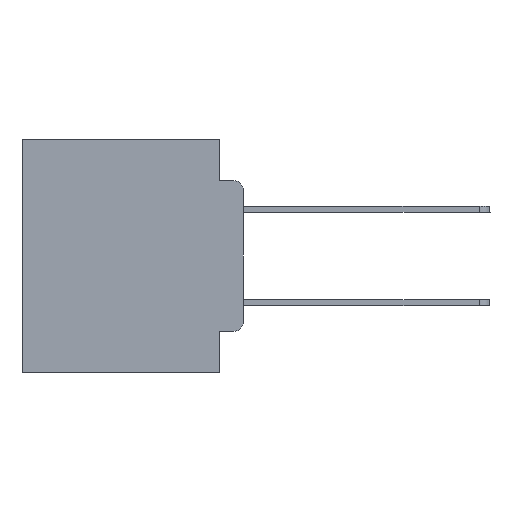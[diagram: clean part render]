
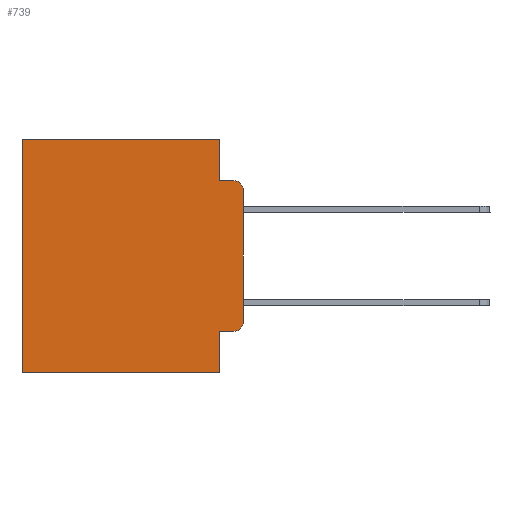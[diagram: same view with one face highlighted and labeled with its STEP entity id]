
A CAD part, left-side view. The second image highlights one B-rep face of the part: STEP entity #739.
In plain terms, the highlighted planar face has unit normal (-1, 0, 0).
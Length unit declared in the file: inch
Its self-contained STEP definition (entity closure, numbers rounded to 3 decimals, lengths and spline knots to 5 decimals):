
#26 = CARTESIAN_POINT ( 'NONE',  ( 0.298, 0.051, -0.0885 ) ) ;
#120 = VECTOR ( 'NONE', #21423, 39.37008 ) ;
#159 = CARTESIAN_POINT ( 'NONE',  ( 0.298, 0., 0. ) ) ;
#609 = DIRECTION ( 'NONE',  ( 1., 0., 0. ) ) ;
#739 = ADVANCED_FACE ( 'NONE', ( #1329 ), #1638, .F. ) ;
#856 = VECTOR ( 'NONE', #21881, 39.37008 ) ;
#1193 = CARTESIAN_POINT ( 'NONE',  ( 0.298, 0., -0.3915 ) ) ;
#1238 = CARTESIAN_POINT ( 'NONE',  ( 0.298, 0.051, -0.0885 ) ) ;
#1329 = FACE_OUTER_BOUND ( 'NONE', #7483, .T. ) ;
#1638 = PLANE ( 'NONE',  #1843 ) ;
#1704 = AXIS2_PLACEMENT_3D ( 'NONE', #23656, #2278, #13862 ) ;
#1843 = AXIS2_PLACEMENT_3D ( 'NONE', #21534, #609, #10963 ) ;
#2278 = DIRECTION ( 'NONE',  ( -1., 0., 0. ) ) ;
#2635 = CARTESIAN_POINT ( 'NONE',  ( 0.298, 0.473, 0. ) ) ;
#3760 = EDGE_CURVE ( 'NONE', #19839, #8971, #24465, .T. ) ;
#4940 = DIRECTION ( 'NONE',  ( 0., 0., -1. ) ) ;
#5090 = CARTESIAN_POINT ( 'NONE',  ( 0.298, 0.473, 0. ) ) ;
#5493 = LINE ( 'NONE', #17071, #21707 ) ;
#6825 = VERTEX_POINT ( 'NONE', #2635 ) ;
#7302 = VERTEX_POINT ( 'NONE', #18890 ) ;
#7483 = EDGE_LOOP ( 'NONE', ( #18309, #27303, #19360, #29055, #19984, #9578, #7896, #28269, #26369, #20470 ) ) ;
#7896 = ORIENTED_EDGE ( 'NONE', *, *, #13026, .F. ) ;
#8004 = LINE ( 'NONE', #5090, #16654 ) ;
#8210 = CARTESIAN_POINT ( 'NONE',  ( 0.298, 0.051, 0. ) ) ;
#8352 = VERTEX_POINT ( 'NONE', #17271 ) ;
#8842 = CARTESIAN_POINT ( 'NONE',  ( 0.298, 0.051, -0.5 ) ) ;
#8971 = VERTEX_POINT ( 'NONE', #1193 ) ;
#9251 = EDGE_CURVE ( 'NONE', #6825, #8352, #8004, .T. ) ;
#9513 = CIRCLE ( 'NONE', #1704, 0.02 ) ;
#9578 = ORIENTED_EDGE ( 'NONE', *, *, #9251, .T. ) ;
#9647 = DIRECTION ( 'NONE',  ( 0., 1., 0. ) ) ;
#10442 = VECTOR ( 'NONE', #26815, 39.37008 ) ;
#10492 = LINE ( 'NONE', #8210, #10442 ) ;
#10567 = DIRECTION ( 'NONE',  ( 0., -1., 0. ) ) ;
#10698 = EDGE_CURVE ( 'NONE', #14037, #19839, #28279, .T. ) ;
#10737 = CARTESIAN_POINT ( 'NONE',  ( 0.298, 0.051, 0. ) ) ;
#10963 = DIRECTION ( 'NONE',  ( 0., 0., -1. ) ) ;
#11614 = VECTOR ( 'NONE', #9647, 39.37008 ) ;
#11631 = LINE ( 'NONE', #159, #11614 ) ;
#11745 = EDGE_CURVE ( 'NONE', #14037, #20097, #10492, .T. ) ;
#11896 = VERTEX_POINT ( 'NONE', #26 ) ;
#12824 = EDGE_CURVE ( 'NONE', #24139, #7302, #9513, .T. ) ;
#13008 = LINE ( 'NONE', #10737, #856 ) ;
#13026 = EDGE_CURVE ( 'NONE', #20097, #8352, #5493, .T. ) ;
#13162 = CARTESIAN_POINT ( 'NONE',  ( 0.298, 0., 0. ) ) ;
#13497 = CARTESIAN_POINT ( 'NONE',  ( 0.298, 0.02, -0.3915 ) ) ;
#13862 = DIRECTION ( 'NONE',  ( 0., 0., -1. ) ) ;
#14037 = VERTEX_POINT ( 'NONE', #21749 ) ;
#14480 = VECTOR ( 'NONE', #10567, 39.37008 ) ;
#15860 = EDGE_CURVE ( 'NONE', #24139, #8971, #25073, .T. ) ;
#16654 = VECTOR ( 'NONE', #4940, 39.37008 ) ;
#17071 = CARTESIAN_POINT ( 'NONE',  ( 0.298, 0., -0.5 ) ) ;
#17271 = CARTESIAN_POINT ( 'NONE',  ( 0.298, 0.473, -0.5 ) ) ;
#17470 = VERTEX_POINT ( 'NONE', #23412 ) ;
#17518 = EDGE_CURVE ( 'NONE', #17470, #6825, #11631, .T. ) ;
#18309 = ORIENTED_EDGE ( 'NONE', *, *, #15860, .F. ) ;
#18527 = DIRECTION ( 'NONE',  ( 0., 0., -1. ) ) ;
#18890 = CARTESIAN_POINT ( 'NONE',  ( 0.298, 0.02, -0.0885 ) ) ;
#19360 = ORIENTED_EDGE ( 'NONE', *, *, #26381, .F. ) ;
#19839 = VERTEX_POINT ( 'NONE', #26249 ) ;
#19984 = ORIENTED_EDGE ( 'NONE', *, *, #17518, .T. ) ;
#20097 = VERTEX_POINT ( 'NONE', #8842 ) ;
#20470 = ORIENTED_EDGE ( 'NONE', *, *, #3760, .T. ) ;
#21267 = CARTESIAN_POINT ( 'NONE',  ( 0.298, 0.051, -0.4115 ) ) ;
#21423 = DIRECTION ( 'NONE',  ( 0., -1., 0. ) ) ;
#21534 = CARTESIAN_POINT ( 'NONE',  ( 0.298, 0., 0. ) ) ;
#21707 = VECTOR ( 'NONE', #28789, 39.37008 ) ;
#21749 = CARTESIAN_POINT ( 'NONE',  ( 0.298, 0.051, -0.4115 ) ) ;
#21881 = DIRECTION ( 'NONE',  ( 0., 0., -1. ) ) ;
#22176 = LINE ( 'NONE', #1238, #14480 ) ;
#22180 = DIRECTION ( 'NONE',  ( 0., 0., -1. ) ) ;
#22567 = CARTESIAN_POINT ( 'NONE',  ( 0.298, 0., -0.1085 ) ) ;
#22828 = DIRECTION ( 'NONE',  ( -1., 0., 0. ) ) ;
#23412 = CARTESIAN_POINT ( 'NONE',  ( 0.298, 0.051, 0. ) ) ;
#23656 = CARTESIAN_POINT ( 'NONE',  ( 0.298, 0.02, -0.1085 ) ) ;
#24139 = VERTEX_POINT ( 'NONE', #22567 ) ;
#24465 = CIRCLE ( 'NONE', #27867, 0.02 ) ;
#25073 = LINE ( 'NONE', #13162, #30028 ) ;
#26249 = CARTESIAN_POINT ( 'NONE',  ( 0.298, 0.02, -0.4115 ) ) ;
#26369 = ORIENTED_EDGE ( 'NONE', *, *, #10698, .T. ) ;
#26381 = EDGE_CURVE ( 'NONE', #11896, #7302, #22176, .T. ) ;
#26815 = DIRECTION ( 'NONE',  ( 0., 0., -1. ) ) ;
#27303 = ORIENTED_EDGE ( 'NONE', *, *, #12824, .T. ) ;
#27696 = EDGE_CURVE ( 'NONE', #17470, #11896, #13008, .T. ) ;
#27867 = AXIS2_PLACEMENT_3D ( 'NONE', #13497, #22828, #18527 ) ;
#28269 = ORIENTED_EDGE ( 'NONE', *, *, #11745, .F. ) ;
#28279 = LINE ( 'NONE', #21267, #120 ) ;
#28789 = DIRECTION ( 'NONE',  ( 0., 1., 0. ) ) ;
#29055 = ORIENTED_EDGE ( 'NONE', *, *, #27696, .F. ) ;
#30028 = VECTOR ( 'NONE', #22180, 39.37008 ) ;
